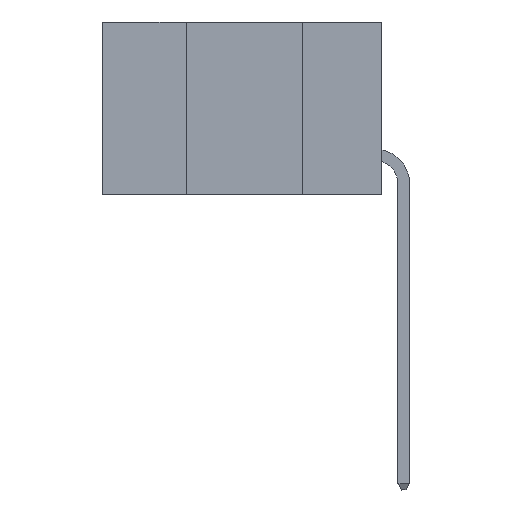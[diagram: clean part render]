
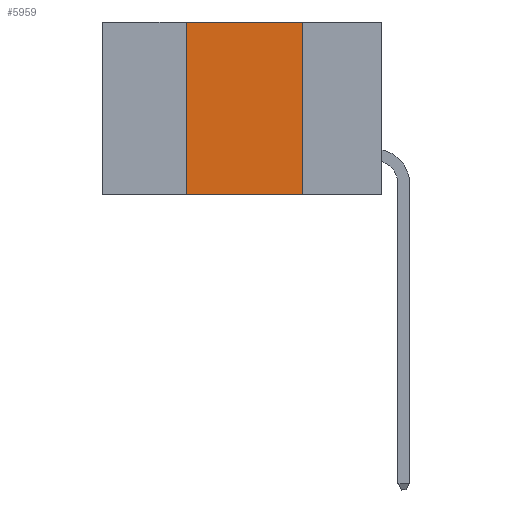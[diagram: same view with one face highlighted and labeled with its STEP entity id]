
A CAD part, left-side view. The second image highlights one B-rep face of the part: STEP entity #5959.
In plain terms, the highlighted planar face has unit normal (-1, 0, 0).
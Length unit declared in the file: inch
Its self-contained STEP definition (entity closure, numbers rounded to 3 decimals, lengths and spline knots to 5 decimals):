
#68 = VERTEX_POINT ( 'NONE', #12681 ) ;
#457 = LINE ( 'NONE', #12076, #12529 ) ;
#472 = EDGE_CURVE ( 'NONE', #3411, #68, #6714, .T. ) ;
#2998 = VECTOR ( 'NONE', #6941, 39.37008 ) ;
#3242 = VERTEX_POINT ( 'NONE', #4254 ) ;
#3411 = VERTEX_POINT ( 'NONE', #8772 ) ;
#3574 = ORIENTED_EDGE ( 'NONE', *, *, #7713, .T. ) ;
#4164 = ORIENTED_EDGE ( 'NONE', *, *, #17988, .F. ) ;
#4254 = CARTESIAN_POINT ( 'NONE',  ( 0., 0.42, 0. ) ) ;
#4257 = CARTESIAN_POINT ( 'NONE',  ( 0., 0.17, 0. ) ) ;
#4436 = AXIS2_PLACEMENT_3D ( 'NONE', #6330, #17634, #10562 ) ;
#5959 = ADVANCED_FACE ( 'NONE', ( #6195 ), #11926, .F. ) ;
#6135 = CARTESIAN_POINT ( 'NONE',  ( 0., 0.6, -0.37 ) ) ;
#6195 = FACE_OUTER_BOUND ( 'NONE', #12743, .T. ) ;
#6330 = CARTESIAN_POINT ( 'NONE',  ( 0., 0.6, 0. ) ) ;
#6714 = LINE ( 'NONE', #4257, #2998 ) ;
#6941 = DIRECTION ( 'NONE',  ( 0., 0., -1. ) ) ;
#6994 = ORIENTED_EDGE ( 'NONE', *, *, #10257, .F. ) ;
#7525 = CARTESIAN_POINT ( 'NONE',  ( 0., 0.6, 0. ) ) ;
#7713 = EDGE_CURVE ( 'NONE', #17618, #68, #10681, .T. ) ;
#8772 = CARTESIAN_POINT ( 'NONE',  ( 0., 0.17, 0. ) ) ;
#10257 = EDGE_CURVE ( 'NONE', #3242, #3411, #13440, .T. ) ;
#10562 = DIRECTION ( 'NONE',  ( 0., 0., -1. ) ) ;
#10681 = LINE ( 'NONE', #6135, #13995 ) ;
#11926 = PLANE ( 'NONE',  #4436 ) ;
#12076 = CARTESIAN_POINT ( 'NONE',  ( 0., 0.42, 0. ) ) ;
#12529 = VECTOR ( 'NONE', #15108, 39.37008 ) ;
#12681 = CARTESIAN_POINT ( 'NONE',  ( 0., 0.17, -0.37 ) ) ;
#12743 = EDGE_LOOP ( 'NONE', ( #15268, #6994, #4164, #3574 ) ) ;
#13440 = LINE ( 'NONE', #7525, #15432 ) ;
#13839 = CARTESIAN_POINT ( 'NONE',  ( 0., 0.42, -0.37 ) ) ;
#13995 = VECTOR ( 'NONE', #17430, 39.37008 ) ;
#15108 = DIRECTION ( 'NONE',  ( 0., 0., 1. ) ) ;
#15268 = ORIENTED_EDGE ( 'NONE', *, *, #472, .F. ) ;
#15432 = VECTOR ( 'NONE', #17339, 39.37008 ) ;
#17339 = DIRECTION ( 'NONE',  ( 0., -1., 0. ) ) ;
#17430 = DIRECTION ( 'NONE',  ( 0., -1., 0. ) ) ;
#17618 = VERTEX_POINT ( 'NONE', #13839 ) ;
#17634 = DIRECTION ( 'NONE',  ( 1., 0., 0. ) ) ;
#17988 = EDGE_CURVE ( 'NONE', #17618, #3242, #457, .T. ) ;
